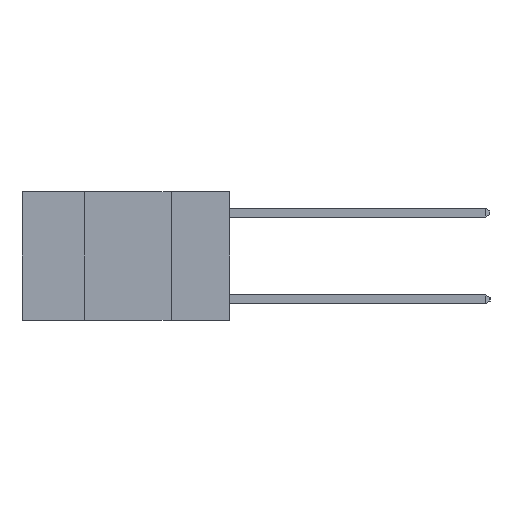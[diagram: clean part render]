
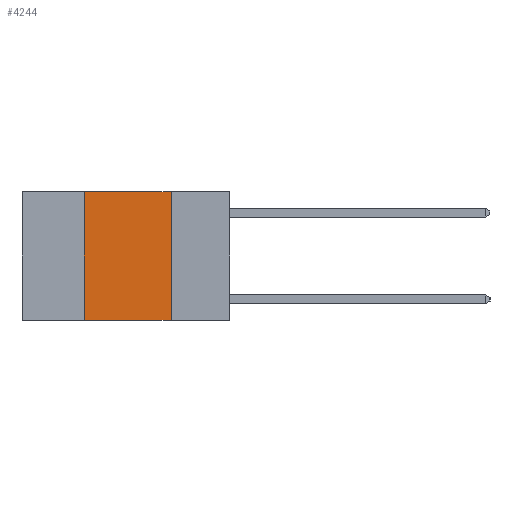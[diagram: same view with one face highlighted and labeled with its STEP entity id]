
A CAD part, left-side view. The second image highlights one B-rep face of the part: STEP entity #4244.
In plain terms, the highlighted planar face has unit normal (-1, 0, 0).
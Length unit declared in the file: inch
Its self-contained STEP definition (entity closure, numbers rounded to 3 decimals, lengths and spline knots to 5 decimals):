
#913 = DIRECTION ( 'NONE',  ( 0., 0., 1. ) ) ;
#1134 = ORIENTED_EDGE ( 'NONE', *, *, #4533, .F. ) ;
#1248 = VECTOR ( 'NONE', #8428, 39.37008 ) ;
#1997 = PLANE ( 'NONE',  #6858 ) ;
#2814 = DIRECTION ( 'NONE',  ( 1., 0., 0. ) ) ;
#3425 = CARTESIAN_POINT ( 'NONE',  ( 0., 0.17, 0. ) ) ;
#3441 = LINE ( 'NONE', #3425, #1248 ) ;
#3740 = LINE ( 'NONE', #10208, #5995 ) ;
#3872 = ORIENTED_EDGE ( 'NONE', *, *, #4251, .T. ) ;
#4244 = ADVANCED_FACE ( 'NONE', ( #10274 ), #1997, .F. ) ;
#4251 = EDGE_CURVE ( 'NONE', #7003, #5544, #3740, .T. ) ;
#4264 = LINE ( 'NONE', #7619, #6261 ) ;
#4378 = CARTESIAN_POINT ( 'NONE',  ( 0., 0.6, 0. ) ) ;
#4533 = EDGE_CURVE ( 'NONE', #7003, #10692, #4264, .T. ) ;
#5178 = VECTOR ( 'NONE', #8543, 39.37008 ) ;
#5191 = CARTESIAN_POINT ( 'NONE',  ( 0., 0.17, 0. ) ) ;
#5327 = DIRECTION ( 'NONE',  ( 0., -1., 0. ) ) ;
#5544 = VERTEX_POINT ( 'NONE', #10074 ) ;
#5568 = EDGE_CURVE ( 'NONE', #10692, #9798, #5703, .T. ) ;
#5703 = LINE ( 'NONE', #4378, #5178 ) ;
#5995 = VECTOR ( 'NONE', #5327, 39.37008 ) ;
#6059 = EDGE_LOOP ( 'NONE', ( #10056, #7534, #1134, #3872 ) ) ;
#6252 = EDGE_CURVE ( 'NONE', #9798, #5544, #3441, .T. ) ;
#6261 = VECTOR ( 'NONE', #913, 39.37008 ) ;
#6858 = AXIS2_PLACEMENT_3D ( 'NONE', #9401, #2814, #8644 ) ;
#7003 = VERTEX_POINT ( 'NONE', #7617 ) ;
#7534 = ORIENTED_EDGE ( 'NONE', *, *, #5568, .F. ) ;
#7617 = CARTESIAN_POINT ( 'NONE',  ( 0., 0.42, -0.37 ) ) ;
#7619 = CARTESIAN_POINT ( 'NONE',  ( 0., 0.42, 0. ) ) ;
#8428 = DIRECTION ( 'NONE',  ( 0., 0., -1. ) ) ;
#8543 = DIRECTION ( 'NONE',  ( 0., -1., 0. ) ) ;
#8644 = DIRECTION ( 'NONE',  ( 0., 0., -1. ) ) ;
#9401 = CARTESIAN_POINT ( 'NONE',  ( 0., 0.6, 0. ) ) ;
#9550 = CARTESIAN_POINT ( 'NONE',  ( 0., 0.42, 0. ) ) ;
#9798 = VERTEX_POINT ( 'NONE', #5191 ) ;
#10056 = ORIENTED_EDGE ( 'NONE', *, *, #6252, .F. ) ;
#10074 = CARTESIAN_POINT ( 'NONE',  ( 0., 0.17, -0.37 ) ) ;
#10208 = CARTESIAN_POINT ( 'NONE',  ( 0., 0.6, -0.37 ) ) ;
#10274 = FACE_OUTER_BOUND ( 'NONE', #6059, .T. ) ;
#10692 = VERTEX_POINT ( 'NONE', #9550 ) ;
